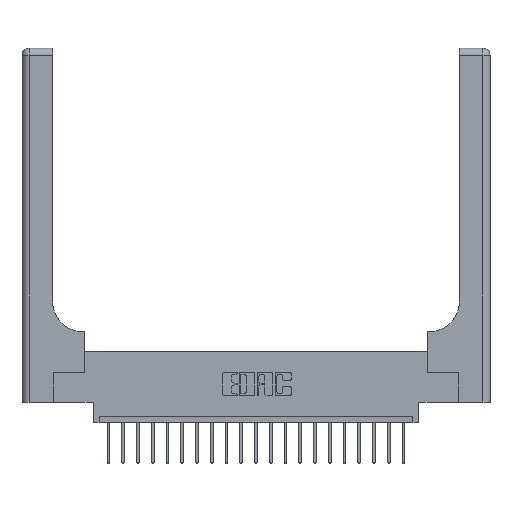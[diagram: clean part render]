
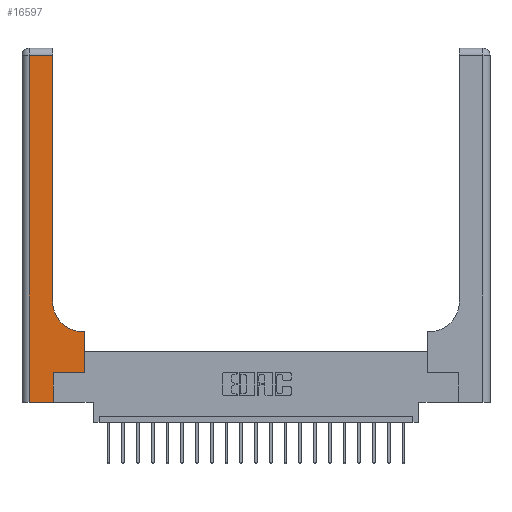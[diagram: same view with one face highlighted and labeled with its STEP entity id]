
A CAD part, top view. The second image highlights one B-rep face of the part: STEP entity #16597.
In plain terms, the highlighted planar face has unit normal (0, 0, 1).
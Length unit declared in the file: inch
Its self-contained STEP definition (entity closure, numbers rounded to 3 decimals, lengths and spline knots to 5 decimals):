
#302 = EDGE_CURVE ( 'NONE', #7670, #1466, #6106, .T. ) ;
#630 = CARTESIAN_POINT ( 'NONE',  ( 0.06, 0., 0.37 ) ) ;
#655 = VECTOR ( 'NONE', #1728, 39.37008 ) ;
#782 = CARTESIAN_POINT ( 'NONE',  ( 0.265, 0.25, 0.37 ) ) ;
#788 = CARTESIAN_POINT ( 'NONE',  ( 0.528, 0.25, 0.37 ) ) ;
#875 = LINE ( 'NONE', #6203, #4166 ) ;
#961 = DIRECTION ( 'NONE',  ( 1., 0., 0. ) ) ;
#1113 = DIRECTION ( 'NONE',  ( -1., 0., 0. ) ) ;
#1466 = VERTEX_POINT ( 'NONE', #10015 ) ;
#1646 = LINE ( 'NONE', #788, #18546 ) ;
#1650 = CARTESIAN_POINT ( 'NONE',  ( 0.06, 2.94, 0.37 ) ) ;
#1728 = DIRECTION ( 'NONE',  ( 0., 1., 0. ) ) ;
#1758 = LINE ( 'NONE', #782, #8173 ) ;
#1773 = DIRECTION ( 'NONE',  ( 1., 0., 0. ) ) ;
#2520 = PLANE ( 'NONE',  #5302 ) ;
#2604 = DIRECTION ( 'NONE',  ( 0., 0., -1. ) ) ;
#3008 = CARTESIAN_POINT ( 'NONE',  ( 0.26, 2.94, 0.37 ) ) ;
#3117 = LINE ( 'NONE', #8930, #20008 ) ;
#3237 = CARTESIAN_POINT ( 'NONE',  ( 0.265, 0., 0.37 ) ) ;
#3396 = EDGE_CURVE ( 'NONE', #13099, #8871, #9046, .T. ) ;
#3549 = VERTEX_POINT ( 'NONE', #3008 ) ;
#3954 = EDGE_CURVE ( 'NONE', #10489, #12720, #1646, .T. ) ;
#4034 = DIRECTION ( 'NONE',  ( 0., 1., 0. ) ) ;
#4100 = ORIENTED_EDGE ( 'NONE', *, *, #4287, .T. ) ;
#4166 = VECTOR ( 'NONE', #1113, 39.37008 ) ;
#4194 = EDGE_LOOP ( 'NONE', ( #9288, #4100, #17447, #5021, #5457, #20863, #12579, #16201, #13811 ) ) ;
#4287 = EDGE_CURVE ( 'NONE', #3549, #13099, #875, .T. ) ;
#4608 = AXIS2_PLACEMENT_3D ( 'NONE', #9201, #18909, #961 ) ;
#5021 = ORIENTED_EDGE ( 'NONE', *, *, #14477, .T. ) ;
#5302 = AXIS2_PLACEMENT_3D ( 'NONE', #14171, #2604, #17436 ) ;
#5457 = ORIENTED_EDGE ( 'NONE', *, *, #9937, .T. ) ;
#6015 = EDGE_CURVE ( 'NONE', #1466, #3549, #6447, .T. ) ;
#6106 = CIRCLE ( 'NONE', #4608, 0.25 ) ;
#6203 = CARTESIAN_POINT ( 'NONE',  ( 0., 2.94, 0.37 ) ) ;
#6267 = CARTESIAN_POINT ( 'NONE',  ( 0.265, 0.25, 0.37 ) ) ;
#6447 = LINE ( 'NONE', #7250, #20782 ) ;
#6585 = EDGE_CURVE ( 'NONE', #12720, #7670, #3117, .T. ) ;
#6864 = CARTESIAN_POINT ( 'NONE',  ( 0.528, 0.6, 0.37 ) ) ;
#7093 = DIRECTION ( 'NONE',  ( 0., -1., 0. ) ) ;
#7250 = CARTESIAN_POINT ( 'NONE',  ( 0.26, 3., 0.37 ) ) ;
#7435 = CARTESIAN_POINT ( 'NONE',  ( 0.265, 0., 0.37 ) ) ;
#7670 = VERTEX_POINT ( 'NONE', #11368 ) ;
#8173 = VECTOR ( 'NONE', #14134, 39.37008 ) ;
#8252 = CARTESIAN_POINT ( 'NONE',  ( 0., 0., 0.37 ) ) ;
#8298 = EDGE_CURVE ( 'NONE', #17407, #10489, #1758, .T. ) ;
#8871 = VERTEX_POINT ( 'NONE', #630 ) ;
#8930 = CARTESIAN_POINT ( 'NONE',  ( 0.26, 0.6, 0.37 ) ) ;
#9046 = LINE ( 'NONE', #20442, #18231 ) ;
#9201 = CARTESIAN_POINT ( 'NONE',  ( 0.51, 0.85, 0.37 ) ) ;
#9288 = ORIENTED_EDGE ( 'NONE', *, *, #6015, .T. ) ;
#9937 = EDGE_CURVE ( 'NONE', #14838, #17407, #19854, .T. ) ;
#10015 = CARTESIAN_POINT ( 'NONE',  ( 0.26, 0.85, 0.37 ) ) ;
#10489 = VERTEX_POINT ( 'NONE', #14241 ) ;
#11118 = DIRECTION ( 'NONE',  ( -1., 0., 0. ) ) ;
#11368 = CARTESIAN_POINT ( 'NONE',  ( 0.51, 0.6, 0.37 ) ) ;
#12213 = FACE_OUTER_BOUND ( 'NONE', #4194, .T. ) ;
#12579 = ORIENTED_EDGE ( 'NONE', *, *, #3954, .T. ) ;
#12720 = VERTEX_POINT ( 'NONE', #6864 ) ;
#13099 = VERTEX_POINT ( 'NONE', #1650 ) ;
#13811 = ORIENTED_EDGE ( 'NONE', *, *, #302, .T. ) ;
#14134 = DIRECTION ( 'NONE',  ( 1., 0., 0. ) ) ;
#14145 = VECTOR ( 'NONE', #1773, 39.37008 ) ;
#14171 = CARTESIAN_POINT ( 'NONE',  ( 0., 3., 0.37 ) ) ;
#14241 = CARTESIAN_POINT ( 'NONE',  ( 0.528, 0.25, 0.37 ) ) ;
#14477 = EDGE_CURVE ( 'NONE', #8871, #14838, #20753, .T. ) ;
#14838 = VERTEX_POINT ( 'NONE', #7435 ) ;
#16201 = ORIENTED_EDGE ( 'NONE', *, *, #6585, .T. ) ;
#16597 = ADVANCED_FACE ( 'NONE', ( #12213 ), #2520, .F. ) ;
#17407 = VERTEX_POINT ( 'NONE', #6267 ) ;
#17436 = DIRECTION ( 'NONE',  ( -1., 0., 0. ) ) ;
#17447 = ORIENTED_EDGE ( 'NONE', *, *, #3396, .T. ) ;
#18231 = VECTOR ( 'NONE', #7093, 39.37008 ) ;
#18546 = VECTOR ( 'NONE', #4034, 39.37008 ) ;
#18682 = DIRECTION ( 'NONE',  ( 0., 1., 0. ) ) ;
#18909 = DIRECTION ( 'NONE',  ( 0., 0., -1. ) ) ;
#19854 = LINE ( 'NONE', #3237, #655 ) ;
#20008 = VECTOR ( 'NONE', #11118, 39.37008 ) ;
#20442 = CARTESIAN_POINT ( 'NONE',  ( 0.06, 3., 0.37 ) ) ;
#20753 = LINE ( 'NONE', #8252, #14145 ) ;
#20782 = VECTOR ( 'NONE', #18682, 39.37008 ) ;
#20863 = ORIENTED_EDGE ( 'NONE', *, *, #8298, .T. ) ;
